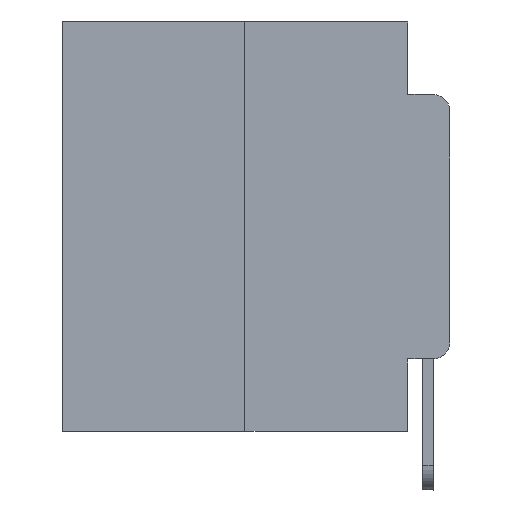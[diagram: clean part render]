
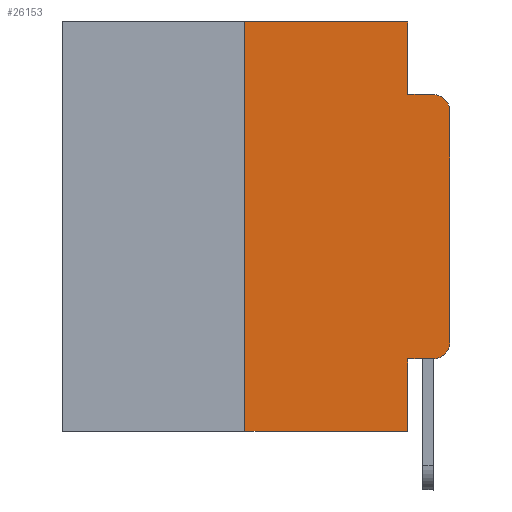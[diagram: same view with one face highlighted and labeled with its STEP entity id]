
A CAD part, left-side view. The second image highlights one B-rep face of the part: STEP entity #26153.
In plain terms, the highlighted planar face has unit normal (-1, 0, 0).
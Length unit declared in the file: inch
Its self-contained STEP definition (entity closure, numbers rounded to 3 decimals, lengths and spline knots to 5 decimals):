
#34 = EDGE_CURVE ( 'NONE', #24701, #3111, #10492, .T. ) ;
#1328 = CARTESIAN_POINT ( 'NONE',  ( 0., 0.02, -0.1085 ) ) ;
#1493 = VECTOR ( 'NONE', #1597, 39.37008 ) ;
#1566 = CARTESIAN_POINT ( 'NONE',  ( 0., 0.02, -0.4115 ) ) ;
#1597 = DIRECTION ( 'NONE',  ( 0., 0., 1. ) ) ;
#2309 = EDGE_CURVE ( 'NONE', #15589, #5271, #16980, .T. ) ;
#2974 = VECTOR ( 'NONE', #3225, 39.37008 ) ;
#3111 = VERTEX_POINT ( 'NONE', #17296 ) ;
#3217 = DIRECTION ( 'NONE',  ( 0., 0., -1. ) ) ;
#3225 = DIRECTION ( 'NONE',  ( 0., 0., -1. ) ) ;
#3915 = DIRECTION ( 'NONE',  ( 0., 0., -1. ) ) ;
#3965 = VECTOR ( 'NONE', #7993, 39.37008 ) ;
#4501 = CARTESIAN_POINT ( 'NONE',  ( 0., 0.051, -0.4115 ) ) ;
#4628 = ORIENTED_EDGE ( 'NONE', *, *, #16991, .T. ) ;
#4675 = AXIS2_PLACEMENT_3D ( 'NONE', #24769, #20326, #12212 ) ;
#5116 = LINE ( 'NONE', #7156, #22768 ) ;
#5271 = VERTEX_POINT ( 'NONE', #24839 ) ;
#5829 = VECTOR ( 'NONE', #25349, 39.37008 ) ;
#6386 = FACE_OUTER_BOUND ( 'NONE', #7095, .T. ) ;
#7095 = EDGE_LOOP ( 'NONE', ( #8764, #22914, #22797, #26075, #19362, #7773, #8293, #13908, #24463, #4628 ) ) ;
#7156 = CARTESIAN_POINT ( 'NONE',  ( 0., 0.051, -0.0885 ) ) ;
#7542 = VECTOR ( 'NONE', #3915, 39.37008 ) ;
#7708 = CARTESIAN_POINT ( 'NONE',  ( 0., 0.051, -0.4115 ) ) ;
#7773 = ORIENTED_EDGE ( 'NONE', *, *, #17284, .F. ) ;
#7993 = DIRECTION ( 'NONE',  ( 0., -1., 0. ) ) ;
#8293 = ORIENTED_EDGE ( 'NONE', *, *, #2309, .T. ) ;
#8387 = LINE ( 'NONE', #22713, #7542 ) ;
#8764 = ORIENTED_EDGE ( 'NONE', *, *, #14288, .T. ) ;
#9583 = LINE ( 'NONE', #23772, #2974 ) ;
#10017 = CARTESIAN_POINT ( 'NONE',  ( 0., 0.473, 0. ) ) ;
#10092 = CARTESIAN_POINT ( 'NONE',  ( 0., 0., -0.3915 ) ) ;
#10454 = EDGE_CURVE ( 'NONE', #21134, #14786, #26484, .T. ) ;
#10492 = CIRCLE ( 'NONE', #25589, 0.02 ) ;
#11161 = CARTESIAN_POINT ( 'NONE',  ( 0., 0.02, -0.3915 ) ) ;
#11927 = VECTOR ( 'NONE', #20735, 39.37008 ) ;
#12212 = DIRECTION ( 'NONE',  ( 0., 0., -1. ) ) ;
#12550 = VERTEX_POINT ( 'NONE', #10092 ) ;
#13074 = DIRECTION ( 'NONE',  ( -1., 0., 0. ) ) ;
#13698 = VERTEX_POINT ( 'NONE', #4501 ) ;
#13770 = VECTOR ( 'NONE', #15958, 39.37008 ) ;
#13908 = ORIENTED_EDGE ( 'NONE', *, *, #15599, .F. ) ;
#14288 = EDGE_CURVE ( 'NONE', #12550, #24701, #17829, .T. ) ;
#14786 = VERTEX_POINT ( 'NONE', #16291 ) ;
#14829 = DIRECTION ( 'NONE',  ( 0., 0., -1. ) ) ;
#15225 = CARTESIAN_POINT ( 'NONE',  ( 0., 0.473, -0.5 ) ) ;
#15589 = VERTEX_POINT ( 'NONE', #16360 ) ;
#15599 = EDGE_CURVE ( 'NONE', #13698, #5271, #8387, .T. ) ;
#15958 = DIRECTION ( 'NONE',  ( 0., -1., 0. ) ) ;
#16291 = CARTESIAN_POINT ( 'NONE',  ( 0., 0.051, 0. ) ) ;
#16360 = CARTESIAN_POINT ( 'NONE',  ( 0., 0.25, -0.5 ) ) ;
#16652 = CARTESIAN_POINT ( 'NONE',  ( 0., 0.25, 0. ) ) ;
#16980 = LINE ( 'NONE', #15225, #5829 ) ;
#16991 = EDGE_CURVE ( 'NONE', #25689, #12550, #17544, .T. ) ;
#17284 = EDGE_CURVE ( 'NONE', #15589, #21134, #22634, .T. ) ;
#17296 = CARTESIAN_POINT ( 'NONE',  ( 0., 0.02, -0.0885 ) ) ;
#17436 = CARTESIAN_POINT ( 'NONE',  ( 0., 0.051, -0.0885 ) ) ;
#17544 = CIRCLE ( 'NONE', #22274, 0.02 ) ;
#17829 = LINE ( 'NONE', #26311, #1493 ) ;
#18329 = CARTESIAN_POINT ( 'NONE',  ( 0., 0.25, 0. ) ) ;
#18485 = CARTESIAN_POINT ( 'NONE',  ( 0., 0., -0.1085 ) ) ;
#19362 = ORIENTED_EDGE ( 'NONE', *, *, #10454, .F. ) ;
#20326 = DIRECTION ( 'NONE',  ( 1., 0., 0. ) ) ;
#20735 = DIRECTION ( 'NONE',  ( 0., 0., 1. ) ) ;
#21134 = VERTEX_POINT ( 'NONE', #16652 ) ;
#21421 = EDGE_CURVE ( 'NONE', #13698, #25689, #22444, .T. ) ;
#21574 = EDGE_CURVE ( 'NONE', #14786, #21633, #9583, .T. ) ;
#21633 = VERTEX_POINT ( 'NONE', #17436 ) ;
#21738 = DIRECTION ( 'NONE',  ( -1., 0., 0. ) ) ;
#22274 = AXIS2_PLACEMENT_3D ( 'NONE', #11161, #13074, #14829 ) ;
#22444 = LINE ( 'NONE', #7708, #13770 ) ;
#22618 = PLANE ( 'NONE',  #4675 ) ;
#22634 = LINE ( 'NONE', #18329, #11927 ) ;
#22713 = CARTESIAN_POINT ( 'NONE',  ( 0., 0.051, 0. ) ) ;
#22768 = VECTOR ( 'NONE', #25662, 39.37008 ) ;
#22797 = ORIENTED_EDGE ( 'NONE', *, *, #25058, .F. ) ;
#22914 = ORIENTED_EDGE ( 'NONE', *, *, #34, .T. ) ;
#23772 = CARTESIAN_POINT ( 'NONE',  ( 0., 0.051, 0. ) ) ;
#24463 = ORIENTED_EDGE ( 'NONE', *, *, #21421, .T. ) ;
#24701 = VERTEX_POINT ( 'NONE', #18485 ) ;
#24769 = CARTESIAN_POINT ( 'NONE',  ( 0., 0.473, 0. ) ) ;
#24839 = CARTESIAN_POINT ( 'NONE',  ( 0., 0.051, -0.5 ) ) ;
#25058 = EDGE_CURVE ( 'NONE', #21633, #3111, #5116, .T. ) ;
#25349 = DIRECTION ( 'NONE',  ( 0., -1., 0. ) ) ;
#25589 = AXIS2_PLACEMENT_3D ( 'NONE', #1328, #21738, #3217 ) ;
#25662 = DIRECTION ( 'NONE',  ( 0., -1., 0. ) ) ;
#25689 = VERTEX_POINT ( 'NONE', #1566 ) ;
#26075 = ORIENTED_EDGE ( 'NONE', *, *, #21574, .F. ) ;
#26153 = ADVANCED_FACE ( 'NONE', ( #6386 ), #22618, .F. ) ;
#26311 = CARTESIAN_POINT ( 'NONE',  ( 0., 0., 0. ) ) ;
#26484 = LINE ( 'NONE', #10017, #3965 ) ;
